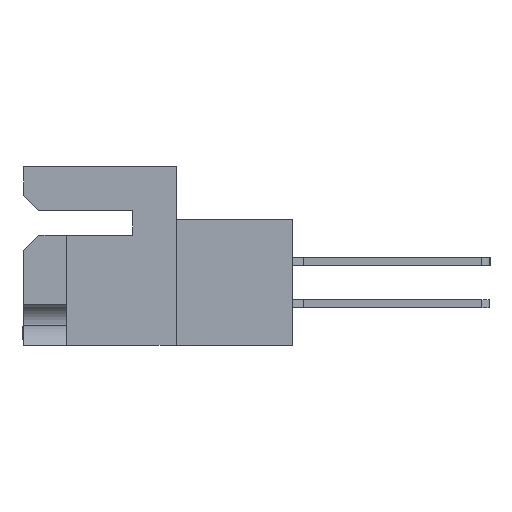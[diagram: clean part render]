
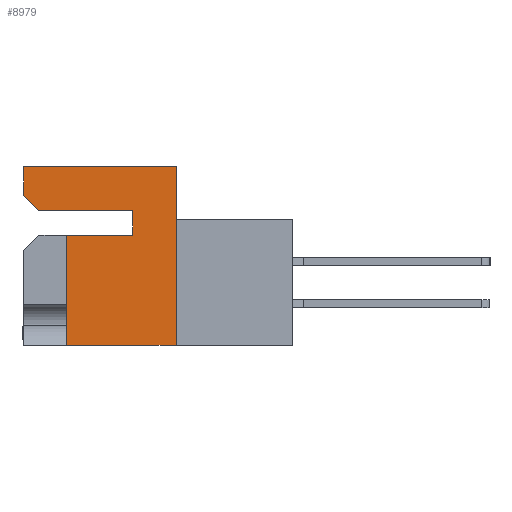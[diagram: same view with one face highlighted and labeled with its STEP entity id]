
A CAD part, left-side view. The second image highlights one B-rep face of the part: STEP entity #8979.
In plain terms, the highlighted planar face has unit normal (-1, 0, 0).
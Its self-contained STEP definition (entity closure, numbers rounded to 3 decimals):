
#2257 = VECTOR ( 'NONE', #29425, 1000. ) ;
#3089 = DIRECTION ( 'NONE',  ( 1., 0., 0. ) ) ;
#3257 = EDGE_CURVE ( 'NONE', #8861, #20620, #18900, .T. ) ;
#3560 = VECTOR ( 'NONE', #15140, 1000. ) ;
#4348 = CARTESIAN_POINT ( 'NONE',  ( 0., 0., -5.182 ) ) ;
#5084 = DIRECTION ( 'NONE',  ( 0., 1., 0. ) ) ;
#5207 = DIRECTION ( 'NONE',  ( 0., -0.707, -0.707 ) ) ;
#5347 = VERTEX_POINT ( 'NONE', #8243 ) ;
#6231 = PLANE ( 'NONE',  #17098 ) ;
#6827 = CARTESIAN_POINT ( 'NONE',  ( 0., 8.255, -5.182 ) ) ;
#6838 = EDGE_CURVE ( 'NONE', #32834, #39762, #30899, .T. ) ;
#8207 = EDGE_CURVE ( 'NONE', #39241, #37239, #26226, .T. ) ;
#8243 = CARTESIAN_POINT ( 'NONE',  ( 0., 0., 0. ) ) ;
#8335 = CARTESIAN_POINT ( 'NONE',  ( 0., -8.814, -13.487 ) ) ;
#8798 = ORIENTED_EDGE ( 'NONE', *, *, #25659, .F. ) ;
#8861 = VERTEX_POINT ( 'NONE', #11523 ) ;
#8979 = ADVANCED_FACE ( 'NONE', ( #9392 ), #6231, .F. ) ;
#9392 = FACE_OUTER_BOUND ( 'NONE', #40080, .T. ) ;
#9898 = LINE ( 'NONE', #21239, #3560 ) ;
#11523 = CARTESIAN_POINT ( 'NONE',  ( 0., 8.255, -5.182 ) ) ;
#12835 = ORIENTED_EDGE ( 'NONE', *, *, #23246, .F. ) ;
#13011 = LINE ( 'NONE', #25339, #34136 ) ;
#15140 = DIRECTION ( 'NONE',  ( 0., -1., 0. ) ) ;
#15508 = ORIENTED_EDGE ( 'NONE', *, *, #3257, .F. ) ;
#15795 = DIRECTION ( 'NONE',  ( 0., 0., -1. ) ) ;
#15837 = DIRECTION ( 'NONE',  ( 0., 0., 1. ) ) ;
#16749 = ORIENTED_EDGE ( 'NONE', *, *, #28215, .F. ) ;
#16783 = CARTESIAN_POINT ( 'NONE',  ( 0., 11.506, -13.487 ) ) ;
#16791 = ORIENTED_EDGE ( 'NONE', *, *, #26401, .F. ) ;
#17098 = AXIS2_PLACEMENT_3D ( 'NONE', #37732, #3089, #15795 ) ;
#17247 = ORIENTED_EDGE ( 'NONE', *, *, #31816, .F. ) ;
#18741 = CARTESIAN_POINT ( 'NONE',  ( 0., 8.255, -13.487 ) ) ;
#18900 = LINE ( 'NONE', #4348, #2257 ) ;
#18925 = CARTESIAN_POINT ( 'NONE',  ( 0., 3.251, -3.302 ) ) ;
#19022 = CARTESIAN_POINT ( 'NONE',  ( 0., 0., -13.487 ) ) ;
#19744 = EDGE_CURVE ( 'NONE', #5347, #32834, #38418, .T. ) ;
#20167 = LINE ( 'NONE', #27285, #38803 ) ;
#20620 = VERTEX_POINT ( 'NONE', #23050 ) ;
#20843 = CARTESIAN_POINT ( 'NONE',  ( 0., 10.363, -3.302 ) ) ;
#21239 = CARTESIAN_POINT ( 'NONE',  ( 0., 11.506, 0. ) ) ;
#23050 = CARTESIAN_POINT ( 'NONE',  ( 0., 3.251, -5.182 ) ) ;
#23246 = EDGE_CURVE ( 'NONE', #40680, #37239, #20167, .T. ) ;
#25040 = VERTEX_POINT ( 'NONE', #38103 ) ;
#25339 = CARTESIAN_POINT ( 'NONE',  ( 0., 3.251, -5.182 ) ) ;
#25659 = EDGE_CURVE ( 'NONE', #39241, #25040, #38127, .T. ) ;
#26226 = LINE ( 'NONE', #20843, #29616 ) ;
#26401 = EDGE_CURVE ( 'NONE', #25040, #5347, #9898, .T. ) ;
#26987 = VECTOR ( 'NONE', #39595, 1000. ) ;
#27285 = CARTESIAN_POINT ( 'NONE',  ( 0., 0., -3.302 ) ) ;
#28215 = EDGE_CURVE ( 'NONE', #39762, #8861, #34311, .T. ) ;
#29425 = DIRECTION ( 'NONE',  ( 0., -1., 0. ) ) ;
#29616 = VECTOR ( 'NONE', #5207, 1000. ) ;
#30260 = VECTOR ( 'NONE', #32413, 1000. ) ;
#30522 = ORIENTED_EDGE ( 'NONE', *, *, #19744, .F. ) ;
#30899 = LINE ( 'NONE', #8335, #26987 ) ;
#31816 = EDGE_CURVE ( 'NONE', #20620, #40680, #13011, .T. ) ;
#32413 = DIRECTION ( 'NONE',  ( 0., 0., 1. ) ) ;
#32798 = ORIENTED_EDGE ( 'NONE', *, *, #8207, .T. ) ;
#32834 = VERTEX_POINT ( 'NONE', #19022 ) ;
#32946 = CARTESIAN_POINT ( 'NONE',  ( 0., 0., 0. ) ) ;
#33199 = DIRECTION ( 'NONE',  ( 0., 0., -1. ) ) ;
#34136 = VECTOR ( 'NONE', #15837, 1000. ) ;
#34311 = LINE ( 'NONE', #6827, #37746 ) ;
#35994 = VECTOR ( 'NONE', #33199, 1000. ) ;
#37239 = VERTEX_POINT ( 'NONE', #40227 ) ;
#37415 = CARTESIAN_POINT ( 'NONE',  ( 0., 11.506, -2.159 ) ) ;
#37676 = DIRECTION ( 'NONE',  ( 0., 0., 1. ) ) ;
#37732 = CARTESIAN_POINT ( 'NONE',  ( 0., 0., 0. ) ) ;
#37746 = VECTOR ( 'NONE', #37676, 1000. ) ;
#38103 = CARTESIAN_POINT ( 'NONE',  ( 0., 11.506, 0. ) ) ;
#38127 = LINE ( 'NONE', #16783, #30260 ) ;
#38418 = LINE ( 'NONE', #32946, #35994 ) ;
#38803 = VECTOR ( 'NONE', #5084, 1000. ) ;
#39241 = VERTEX_POINT ( 'NONE', #37415 ) ;
#39595 = DIRECTION ( 'NONE',  ( 0., 1., 0. ) ) ;
#39628 = ORIENTED_EDGE ( 'NONE', *, *, #6838, .F. ) ;
#39762 = VERTEX_POINT ( 'NONE', #18741 ) ;
#40080 = EDGE_LOOP ( 'NONE', ( #39628, #30522, #16791, #8798, #32798, #12835, #17247, #15508, #16749 ) ) ;
#40227 = CARTESIAN_POINT ( 'NONE',  ( 0., 10.363, -3.302 ) ) ;
#40680 = VERTEX_POINT ( 'NONE', #18925 ) ;
